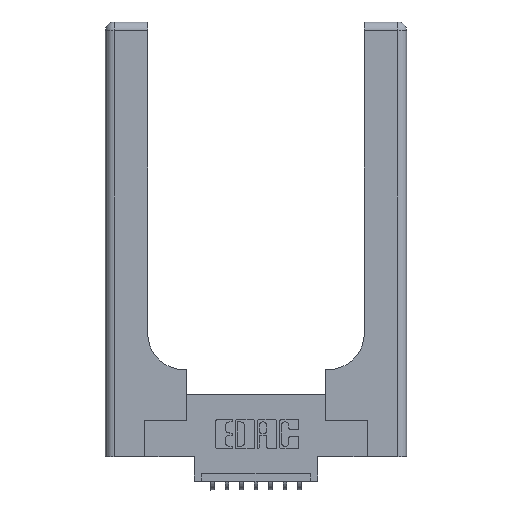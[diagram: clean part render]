
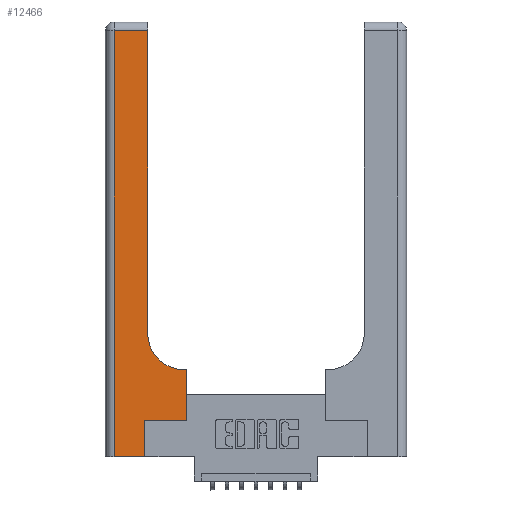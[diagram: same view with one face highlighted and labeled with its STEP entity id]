
A CAD part, top view. The second image highlights one B-rep face of the part: STEP entity #12466.
In plain terms, the highlighted planar face has unit normal (0, 0, 1).
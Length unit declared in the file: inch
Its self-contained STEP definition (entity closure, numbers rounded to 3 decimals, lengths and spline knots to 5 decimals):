
#23 = ORIENTED_EDGE ( 'NONE', *, *, #8933, .T. ) ;
#397 = EDGE_CURVE ( 'NONE', #5601, #7287, #1780, .T. ) ;
#710 = CARTESIAN_POINT ( 'NONE',  ( 0.2915, 2.94, 0.37 ) ) ;
#771 = CARTESIAN_POINT ( 'NONE',  ( 0.5585, 0.6, 0.37 ) ) ;
#975 = CARTESIAN_POINT ( 'NONE',  ( 0.5585, 0.25, 0.37 ) ) ;
#1272 = DIRECTION ( 'NONE',  ( 0., 0., -1. ) ) ;
#1562 = DIRECTION ( 'NONE',  ( -1., 0., 0. ) ) ;
#1780 = LINE ( 'NONE', #14400, #4567 ) ;
#2354 = ORIENTED_EDGE ( 'NONE', *, *, #397, .T. ) ;
#2997 = VERTEX_POINT ( 'NONE', #771 ) ;
#3068 = VECTOR ( 'NONE', #11982, 39.37008 ) ;
#3305 = VERTEX_POINT ( 'NONE', #6285 ) ;
#3403 = CARTESIAN_POINT ( 'NONE',  ( 0.269, 0.25, 0.37 ) ) ;
#3514 = ORIENTED_EDGE ( 'NONE', *, *, #9937, .T. ) ;
#3712 = CARTESIAN_POINT ( 'NONE',  ( 0., 0., 0.37 ) ) ;
#4500 = CARTESIAN_POINT ( 'NONE',  ( 0.06, 3., 0.37 ) ) ;
#4519 = VECTOR ( 'NONE', #9047, 39.37008 ) ;
#4548 = DIRECTION ( 'NONE',  ( -1., 0., 0. ) ) ;
#4567 = VECTOR ( 'NONE', #7353, 39.37008 ) ;
#4592 = VERTEX_POINT ( 'NONE', #9292 ) ;
#4879 = ORIENTED_EDGE ( 'NONE', *, *, #13474, .T. ) ;
#4983 = ORIENTED_EDGE ( 'NONE', *, *, #10078, .T. ) ;
#5057 = LINE ( 'NONE', #4500, #7848 ) ;
#5226 = ORIENTED_EDGE ( 'NONE', *, *, #10670, .T. ) ;
#5601 = VERTEX_POINT ( 'NONE', #14830 ) ;
#5706 = ORIENTED_EDGE ( 'NONE', *, *, #12160, .T. ) ;
#5769 = LINE ( 'NONE', #10755, #10062 ) ;
#5785 = LINE ( 'NONE', #3712, #3068 ) ;
#6116 = CARTESIAN_POINT ( 'NONE',  ( 0., 3., 0.37 ) ) ;
#6285 = CARTESIAN_POINT ( 'NONE',  ( 0.5585, 0.25, 0.37 ) ) ;
#6699 = VERTEX_POINT ( 'NONE', #10917 ) ;
#6776 = VECTOR ( 'NONE', #10448, 39.37008 ) ;
#6820 = VERTEX_POINT ( 'NONE', #10431 ) ;
#6954 = EDGE_LOOP ( 'NONE', ( #2354, #7369, #23, #11019, #5706, #4983, #3514, #4879, #5226 ) ) ;
#7287 = VERTEX_POINT ( 'NONE', #710 ) ;
#7353 = DIRECTION ( 'NONE',  ( 0., 1., 0. ) ) ;
#7369 = ORIENTED_EDGE ( 'NONE', *, *, #8984, .T. ) ;
#7450 = VERTEX_POINT ( 'NONE', #3403 ) ;
#7848 = VECTOR ( 'NONE', #15112, 39.37008 ) ;
#8933 = EDGE_CURVE ( 'NONE', #4592, #6699, #5057, .T. ) ;
#8984 = EDGE_CURVE ( 'NONE', #7287, #4592, #11530, .T. ) ;
#9047 = DIRECTION ( 'NONE',  ( 0., 1., 0. ) ) ;
#9186 = EDGE_CURVE ( 'NONE', #6699, #9715, #5785, .T. ) ;
#9271 = DIRECTION ( 'NONE',  ( 0., 1., 0. ) ) ;
#9292 = CARTESIAN_POINT ( 'NONE',  ( 0.06, 2.94, 0.37 ) ) ;
#9515 = CARTESIAN_POINT ( 'NONE',  ( 0.5415, 0.85, 0.37 ) ) ;
#9562 = PLANE ( 'NONE',  #10131 ) ;
#9715 = VERTEX_POINT ( 'NONE', #11492 ) ;
#9794 = FACE_OUTER_BOUND ( 'NONE', #6954, .T. ) ;
#9937 = EDGE_CURVE ( 'NONE', #3305, #2997, #15072, .T. ) ;
#10062 = VECTOR ( 'NONE', #10704, 39.37008 ) ;
#10078 = EDGE_CURVE ( 'NONE', #7450, #3305, #5769, .T. ) ;
#10131 = AXIS2_PLACEMENT_3D ( 'NONE', #6116, #10928, #1562 ) ;
#10395 = AXIS2_PLACEMENT_3D ( 'NONE', #9515, #1272, #13161 ) ;
#10431 = CARTESIAN_POINT ( 'NONE',  ( 0.5415, 0.6, 0.37 ) ) ;
#10448 = DIRECTION ( 'NONE',  ( -1., 0., 0. ) ) ;
#10621 = VECTOR ( 'NONE', #9271, 39.37008 ) ;
#10670 = EDGE_CURVE ( 'NONE', #6820, #5601, #11686, .T. ) ;
#10704 = DIRECTION ( 'NONE',  ( 1., 0., 0. ) ) ;
#10755 = CARTESIAN_POINT ( 'NONE',  ( 0.269, 0.25, 0.37 ) ) ;
#10917 = CARTESIAN_POINT ( 'NONE',  ( 0.06, 0., 0.37 ) ) ;
#10928 = DIRECTION ( 'NONE',  ( 0., 0., -1. ) ) ;
#11019 = ORIENTED_EDGE ( 'NONE', *, *, #9186, .T. ) ;
#11492 = CARTESIAN_POINT ( 'NONE',  ( 0.269, 0., 0.37 ) ) ;
#11530 = LINE ( 'NONE', #12808, #13196 ) ;
#11559 = CARTESIAN_POINT ( 'NONE',  ( 0.269, 0., 0.37 ) ) ;
#11686 = CIRCLE ( 'NONE', #10395, 0.25 ) ;
#11982 = DIRECTION ( 'NONE',  ( 1., 0., 0. ) ) ;
#12086 = LINE ( 'NONE', #11559, #4519 ) ;
#12160 = EDGE_CURVE ( 'NONE', #9715, #7450, #12086, .T. ) ;
#12466 = ADVANCED_FACE ( 'NONE', ( #9794 ), #9562, .F. ) ;
#12808 = CARTESIAN_POINT ( 'NONE',  ( 0., 2.94, 0.37 ) ) ;
#13161 = DIRECTION ( 'NONE',  ( 1., 0., 0. ) ) ;
#13196 = VECTOR ( 'NONE', #4548, 39.37008 ) ;
#13474 = EDGE_CURVE ( 'NONE', #2997, #6820, #15135, .T. ) ;
#14400 = CARTESIAN_POINT ( 'NONE',  ( 0.2915, 3., 0.37 ) ) ;
#14830 = CARTESIAN_POINT ( 'NONE',  ( 0.2915, 0.85, 0.37 ) ) ;
#15070 = CARTESIAN_POINT ( 'NONE',  ( 0.2915, 0.6, 0.37 ) ) ;
#15072 = LINE ( 'NONE', #975, #10621 ) ;
#15112 = DIRECTION ( 'NONE',  ( 0., -1., 0. ) ) ;
#15135 = LINE ( 'NONE', #15070, #6776 ) ;
